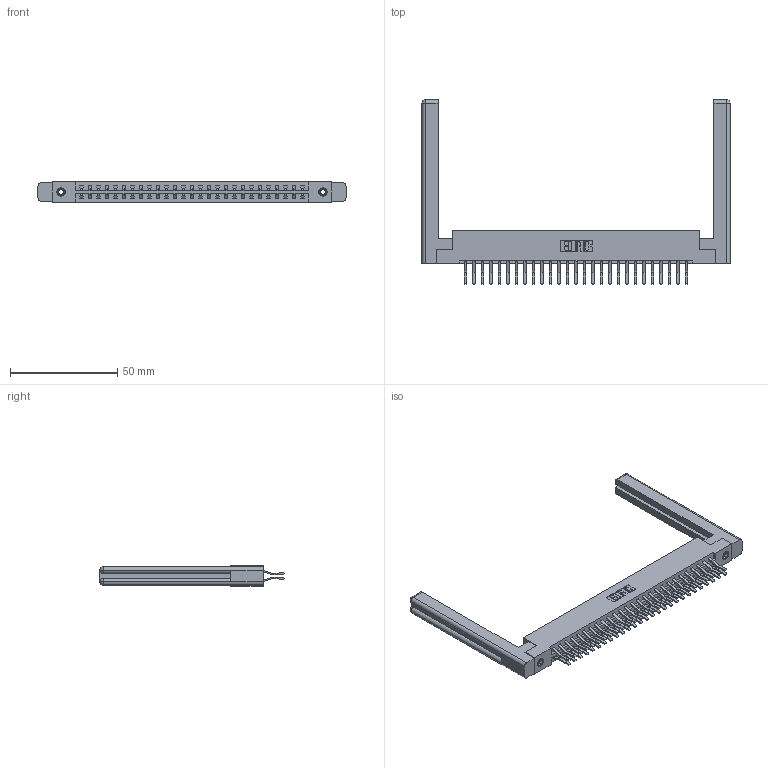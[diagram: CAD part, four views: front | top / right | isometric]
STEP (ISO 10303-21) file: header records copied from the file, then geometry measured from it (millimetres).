
FILE_DESCRIPTION (( 'STEP AP203' ), '1' );
FILE_NAME ('337-054-560-258.STEP', '2019-10-09T18:42:45', ( '' ), ( '' ), 'SwSTEP 2.0', 'SolidWorks 2016', '' );
FILE_SCHEMA (( 'CONFIG_CONTROL_DESIGN' ));
Length unit declared in the file: inch
Products named in the file (5): 345-250-001_345-250-001-102; 307-220-058; 337-054-560-258; 345-292-001_560 Tail; 337 Part_Flush Mounting Lugs - 0.156 Dia-TI
Assembly tree (59 placements, depth 2):
  337-054-560-258
    337 Part_Flush Mounting Lugs - 0.156 Dia-TI
    345-292-001_560 Tail  x54
    345-250-001_345-250-001-102  x2
    307-220-058  x2
Bounding box: 143.61 x 85.87 x 9.4 mm (x, y, z)
Volume: 22431.6 mm3; surface area: 23209.9 mm2
Topology: 59 solids, 59 shells, 3280 faces, 9683 edges, 6370 vertices
Faces by surface type: plane 2206, cylinder 1050, cone 12, torus 12
Entity records: 25596 total; most frequent: CARTESIAN_POINT 4333, ORIENTED_EDGE 4208, DIRECTION 3732, EDGE_CURVE 2104, LINE 1924, VECTOR 1924, VERTEX_POINT 1394, AXIS2_PLACEMENT_3D 904
